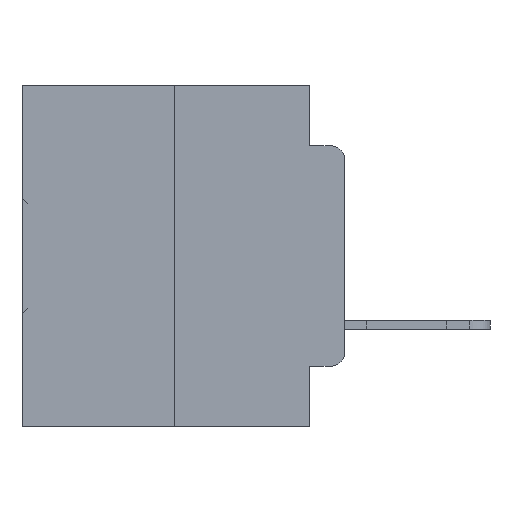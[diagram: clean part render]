
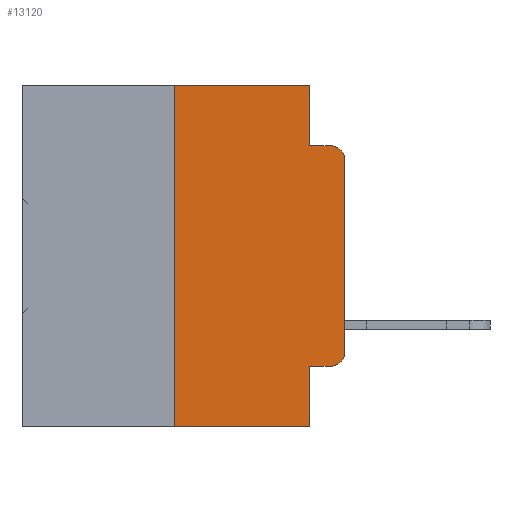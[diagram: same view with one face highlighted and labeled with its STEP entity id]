
A CAD part, left-side view. The second image highlights one B-rep face of the part: STEP entity #13120.
In plain terms, the highlighted planar face has unit normal (-1, 0, 0).
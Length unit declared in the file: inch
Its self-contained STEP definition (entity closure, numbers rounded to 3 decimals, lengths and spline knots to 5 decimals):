
#1474 = EDGE_CURVE ( 'NONE', #2815, #22040, #3344, .T. ) ;
#2288 = ORIENTED_EDGE ( 'NONE', *, *, #18492, .T. ) ;
#2673 = ORIENTED_EDGE ( 'NONE', *, *, #11209, .F. ) ;
#2815 = VERTEX_POINT ( 'NONE', #30729 ) ;
#3344 = LINE ( 'NONE', #19664, #25253 ) ;
#4207 = ORIENTED_EDGE ( 'NONE', *, *, #5475, .F. ) ;
#5475 = EDGE_CURVE ( 'NONE', #31020, #26166, #7365, .T. ) ;
#6151 = DIRECTION ( 'NONE',  ( 0., -1., 0. ) ) ;
#6191 = CARTESIAN_POINT ( 'NONE',  ( 0., 0.051, -0.0885 ) ) ;
#7365 = LINE ( 'NONE', #15354, #22614 ) ;
#7462 = EDGE_CURVE ( 'NONE', #13093, #22015, #27673, .T. ) ;
#7991 = VERTEX_POINT ( 'NONE', #29019 ) ;
#8823 = CIRCLE ( 'NONE', #27136, 0.02 ) ;
#8860 = DIRECTION ( 'NONE',  ( 0., 0., -1. ) ) ;
#8978 = DIRECTION ( 'NONE',  ( 1., 0., 0. ) ) ;
#9337 = EDGE_LOOP ( 'NONE', ( #2288, #10364, #2673, #10750, #29821, #4207, #11221, #20795, #21311, #18488 ) ) ;
#9365 = CARTESIAN_POINT ( 'NONE',  ( 0., 0.473, 0. ) ) ;
#9479 = PLANE ( 'NONE',  #17335 ) ;
#9831 = FACE_OUTER_BOUND ( 'NONE', #9337, .T. ) ;
#10031 = CARTESIAN_POINT ( 'NONE',  ( 0., 0.051, 0. ) ) ;
#10338 = DIRECTION ( 'NONE',  ( -1., 0., 0. ) ) ;
#10364 = ORIENTED_EDGE ( 'NONE', *, *, #14903, .T. ) ;
#10750 = ORIENTED_EDGE ( 'NONE', *, *, #7462, .F. ) ;
#10866 = LINE ( 'NONE', #12114, #30726 ) ;
#11209 = EDGE_CURVE ( 'NONE', #22015, #19898, #22233, .T. ) ;
#11221 = ORIENTED_EDGE ( 'NONE', *, *, #20414, .T. ) ;
#11253 = CARTESIAN_POINT ( 'NONE',  ( 0., 0., 0. ) ) ;
#11476 = DIRECTION ( 'NONE',  ( 0., 0., 1. ) ) ;
#11799 = DIRECTION ( 'NONE',  ( 0., -1., 0. ) ) ;
#11962 = CARTESIAN_POINT ( 'NONE',  ( 0., 0.473, -0.5 ) ) ;
#12114 = CARTESIAN_POINT ( 'NONE',  ( 0., 0.473, 0. ) ) ;
#13047 = VECTOR ( 'NONE', #11799, 39.37008 ) ;
#13093 = VERTEX_POINT ( 'NONE', #10031 ) ;
#13120 = ADVANCED_FACE ( 'NONE', ( #9831 ), #9479, .F. ) ;
#13353 = CARTESIAN_POINT ( 'NONE',  ( 0., 0.051, 0. ) ) ;
#14544 = LINE ( 'NONE', #11253, #33801 ) ;
#14903 = EDGE_CURVE ( 'NONE', #7991, #19898, #8823, .T. ) ;
#15354 = CARTESIAN_POINT ( 'NONE',  ( 0., 0.25, 0. ) ) ;
#15571 = CARTESIAN_POINT ( 'NONE',  ( 0., 0.051, 0. ) ) ;
#15998 = EDGE_CURVE ( 'NONE', #26166, #13093, #10866, .T. ) ;
#17335 = AXIS2_PLACEMENT_3D ( 'NONE', #9365, #8978, #8860 ) ;
#18488 = ORIENTED_EDGE ( 'NONE', *, *, #30923, .T. ) ;
#18492 = EDGE_CURVE ( 'NONE', #18557, #7991, #14544, .T. ) ;
#18557 = VERTEX_POINT ( 'NONE', #32963 ) ;
#19039 = DIRECTION ( 'NONE',  ( 0., -1., 0. ) ) ;
#19142 = DIRECTION ( 'NONE',  ( 0., 0., 1. ) ) ;
#19664 = CARTESIAN_POINT ( 'NONE',  ( 0., 0.051, -0.4115 ) ) ;
#19898 = VERTEX_POINT ( 'NONE', #30928 ) ;
#20234 = DIRECTION ( 'NONE',  ( 0., -1., 0. ) ) ;
#20414 = EDGE_CURVE ( 'NONE', #31020, #21395, #33268, .T. ) ;
#20482 = CARTESIAN_POINT ( 'NONE',  ( 0., 0.051, -0.5 ) ) ;
#20795 = ORIENTED_EDGE ( 'NONE', *, *, #34034, .F. ) ;
#20852 = VECTOR ( 'NONE', #30339, 39.37008 ) ;
#21311 = ORIENTED_EDGE ( 'NONE', *, *, #1474, .T. ) ;
#21395 = VERTEX_POINT ( 'NONE', #20482 ) ;
#22015 = VERTEX_POINT ( 'NONE', #30230 ) ;
#22040 = VERTEX_POINT ( 'NONE', #30699 ) ;
#22233 = LINE ( 'NONE', #6191, #32939 ) ;
#22327 = CIRCLE ( 'NONE', #31628, 0.02 ) ;
#22614 = VECTOR ( 'NONE', #11476, 39.37008 ) ;
#24619 = DIRECTION ( 'NONE',  ( 0., 0., -1. ) ) ;
#24729 = DIRECTION ( 'NONE',  ( -1., 0., 0. ) ) ;
#24731 = CARTESIAN_POINT ( 'NONE',  ( 0., 0.02, -0.1085 ) ) ;
#25047 = CARTESIAN_POINT ( 'NONE',  ( 0., 0.25, 0. ) ) ;
#25253 = VECTOR ( 'NONE', #20234, 39.37008 ) ;
#26166 = VERTEX_POINT ( 'NONE', #25047 ) ;
#26252 = CARTESIAN_POINT ( 'NONE',  ( 0., 0.02, -0.3915 ) ) ;
#27136 = AXIS2_PLACEMENT_3D ( 'NONE', #24731, #24729, #24619 ) ;
#27538 = VECTOR ( 'NONE', #33193, 39.37008 ) ;
#27673 = LINE ( 'NONE', #13353, #20852 ) ;
#28690 = DIRECTION ( 'NONE',  ( 0., 0., -1. ) ) ;
#29019 = CARTESIAN_POINT ( 'NONE',  ( 0., 0., -0.1085 ) ) ;
#29754 = LINE ( 'NONE', #15571, #27538 ) ;
#29821 = ORIENTED_EDGE ( 'NONE', *, *, #15998, .F. ) ;
#30230 = CARTESIAN_POINT ( 'NONE',  ( 0., 0.051, -0.0885 ) ) ;
#30339 = DIRECTION ( 'NONE',  ( 0., 0., -1. ) ) ;
#30699 = CARTESIAN_POINT ( 'NONE',  ( 0., 0.02, -0.4115 ) ) ;
#30726 = VECTOR ( 'NONE', #19039, 39.37008 ) ;
#30729 = CARTESIAN_POINT ( 'NONE',  ( 0., 0.051, -0.4115 ) ) ;
#30923 = EDGE_CURVE ( 'NONE', #22040, #18557, #22327, .T. ) ;
#30928 = CARTESIAN_POINT ( 'NONE',  ( 0., 0.02, -0.0885 ) ) ;
#31020 = VERTEX_POINT ( 'NONE', #34026 ) ;
#31628 = AXIS2_PLACEMENT_3D ( 'NONE', #26252, #10338, #28690 ) ;
#32939 = VECTOR ( 'NONE', #6151, 39.37008 ) ;
#32963 = CARTESIAN_POINT ( 'NONE',  ( 0., 0., -0.3915 ) ) ;
#33193 = DIRECTION ( 'NONE',  ( 0., 0., -1. ) ) ;
#33268 = LINE ( 'NONE', #11962, #13047 ) ;
#33801 = VECTOR ( 'NONE', #19142, 39.37008 ) ;
#34026 = CARTESIAN_POINT ( 'NONE',  ( 0., 0.25, -0.5 ) ) ;
#34034 = EDGE_CURVE ( 'NONE', #2815, #21395, #29754, .T. ) ;
